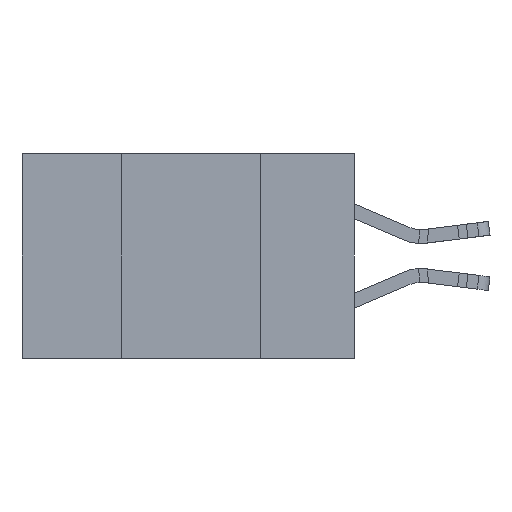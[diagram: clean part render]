
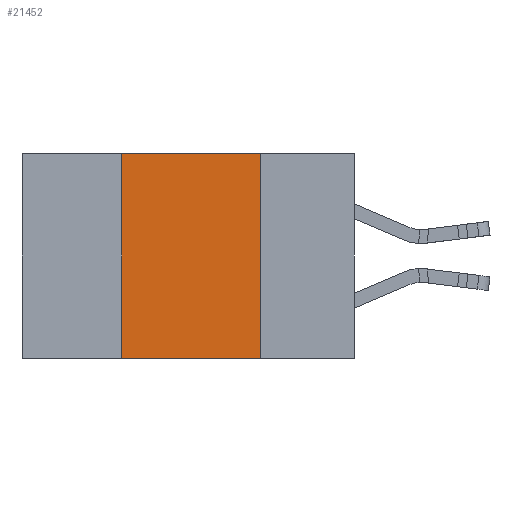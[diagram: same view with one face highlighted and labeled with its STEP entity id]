
A CAD part, left-side view. The second image highlights one B-rep face of the part: STEP entity #21452.
In plain terms, the highlighted planar face has unit normal (-1, 0, 0).
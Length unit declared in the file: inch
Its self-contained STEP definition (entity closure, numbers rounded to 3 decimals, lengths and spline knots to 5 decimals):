
#445 = PLANE ( 'NONE',  #18152 ) ;
#2317 = CARTESIAN_POINT ( 'NONE',  ( 0., 0.17, -0.37 ) ) ;
#3446 = CARTESIAN_POINT ( 'NONE',  ( 0., 0.6, 0. ) ) ;
#7445 = CARTESIAN_POINT ( 'NONE',  ( 0., 0.42, -0.37 ) ) ;
#7573 = ORIENTED_EDGE ( 'NONE', *, *, #12773, .F. ) ;
#7910 = CARTESIAN_POINT ( 'NONE',  ( 0., 0.17, -0.37 ) ) ;
#8667 = VECTOR ( 'NONE', #25032, 39.37008 ) ;
#8745 = EDGE_CURVE ( 'NONE', #9355, #11668, #20717, .T. ) ;
#8833 = VERTEX_POINT ( 'NONE', #13199 ) ;
#9355 = VERTEX_POINT ( 'NONE', #19752 ) ;
#9401 = VECTOR ( 'NONE', #11304, 39.37008 ) ;
#10156 = DIRECTION ( 'NONE',  ( 0., 0., -1. ) ) ;
#10320 = DIRECTION ( 'NONE',  ( 1., 0., 0. ) ) ;
#11153 = EDGE_CURVE ( 'NONE', #8833, #22302, #21122, .T. ) ;
#11304 = DIRECTION ( 'NONE',  ( 0., -1., 0. ) ) ;
#11668 = VERTEX_POINT ( 'NONE', #7910 ) ;
#11811 = VECTOR ( 'NONE', #15143, 39.37008 ) ;
#12076 = LINE ( 'NONE', #2317, #17679 ) ;
#12239 = CARTESIAN_POINT ( 'NONE',  ( 0., 0.6, 0. ) ) ;
#12773 = EDGE_CURVE ( 'NONE', #22302, #11668, #12076, .T. ) ;
#13068 = CARTESIAN_POINT ( 'NONE',  ( 0., 0.6, -0.37 ) ) ;
#13199 = CARTESIAN_POINT ( 'NONE',  ( 0., 0.42, 0. ) ) ;
#15143 = DIRECTION ( 'NONE',  ( 0., -1., 0. ) ) ;
#16944 = ORIENTED_EDGE ( 'NONE', *, *, #8745, .T. ) ;
#17679 = VECTOR ( 'NONE', #10156, 39.37008 ) ;
#17953 = FACE_OUTER_BOUND ( 'NONE', #19728, .T. ) ;
#18152 = AXIS2_PLACEMENT_3D ( 'NONE', #12239, #10320, #19758 ) ;
#19728 = EDGE_LOOP ( 'NONE', ( #7573, #19818, #24413, #16944 ) ) ;
#19752 = CARTESIAN_POINT ( 'NONE',  ( 0., 0.42, -0.37 ) ) ;
#19758 = DIRECTION ( 'NONE',  ( 0., 0., -1. ) ) ;
#19818 = ORIENTED_EDGE ( 'NONE', *, *, #11153, .F. ) ;
#20717 = LINE ( 'NONE', #13068, #11811 ) ;
#21122 = LINE ( 'NONE', #3446, #9401 ) ;
#21452 = ADVANCED_FACE ( 'NONE', ( #17953 ), #445, .F. ) ;
#22219 = EDGE_CURVE ( 'NONE', #9355, #8833, #23224, .T. ) ;
#22302 = VERTEX_POINT ( 'NONE', #22968 ) ;
#22968 = CARTESIAN_POINT ( 'NONE',  ( 0., 0.17, 0. ) ) ;
#23224 = LINE ( 'NONE', #7445, #8667 ) ;
#24413 = ORIENTED_EDGE ( 'NONE', *, *, #22219, .F. ) ;
#25032 = DIRECTION ( 'NONE',  ( 0., 0., 1. ) ) ;
